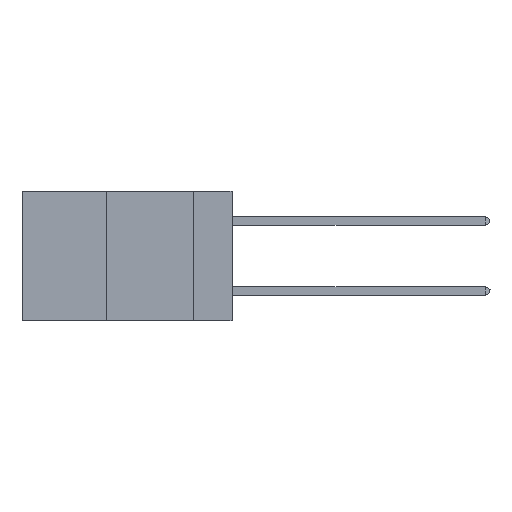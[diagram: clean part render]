
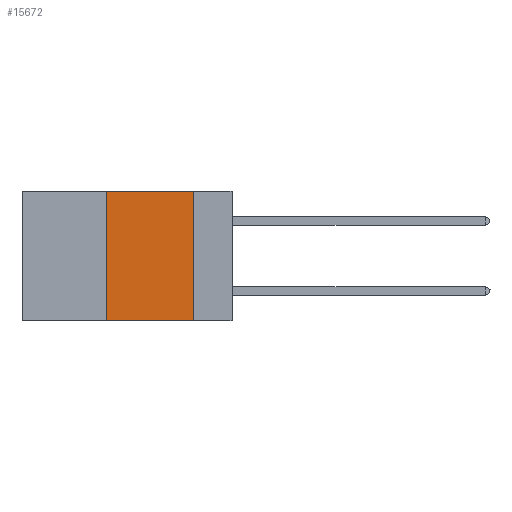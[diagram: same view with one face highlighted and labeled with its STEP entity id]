
A CAD part, left-side view. The second image highlights one B-rep face of the part: STEP entity #15672.
In plain terms, the highlighted planar face has unit normal (-1, 0, 0).
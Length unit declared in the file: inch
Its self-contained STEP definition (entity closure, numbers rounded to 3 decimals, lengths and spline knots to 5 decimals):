
#321 = PLANE ( 'NONE',  #1953 ) ;
#846 = VECTOR ( 'NONE', #3519, 39.37008 ) ;
#1703 = CARTESIAN_POINT ( 'NONE',  ( 0., 0.11, 0. ) ) ;
#1807 = VERTEX_POINT ( 'NONE', #18376 ) ;
#1953 = AXIS2_PLACEMENT_3D ( 'NONE', #6046, #10335, #5559 ) ;
#2399 = FACE_OUTER_BOUND ( 'NONE', #6142, .T. ) ;
#2814 = EDGE_CURVE ( 'NONE', #11081, #12556, #5614, .T. ) ;
#3041 = ORIENTED_EDGE ( 'NONE', *, *, #2814, .F. ) ;
#3519 = DIRECTION ( 'NONE',  ( 0., -1., 0. ) ) ;
#4513 = VECTOR ( 'NONE', #21857, 39.37008 ) ;
#4859 = LINE ( 'NONE', #13328, #4513 ) ;
#5559 = DIRECTION ( 'NONE',  ( 0., 0., -1. ) ) ;
#5614 = LINE ( 'NONE', #1703, #26925 ) ;
#5883 = ORIENTED_EDGE ( 'NONE', *, *, #22800, .F. ) ;
#6046 = CARTESIAN_POINT ( 'NONE',  ( 0., 0.6, 0. ) ) ;
#6142 = EDGE_LOOP ( 'NONE', ( #3041, #5883, #9761, #21176 ) ) ;
#7833 = DIRECTION ( 'NONE',  ( 0., 0., -1. ) ) ;
#9761 = ORIENTED_EDGE ( 'NONE', *, *, #15770, .F. ) ;
#10335 = DIRECTION ( 'NONE',  ( 1., 0., 0. ) ) ;
#11081 = VERTEX_POINT ( 'NONE', #18260 ) ;
#12556 = VERTEX_POINT ( 'NONE', #13640 ) ;
#12992 = EDGE_CURVE ( 'NONE', #1807, #12556, #4859, .T. ) ;
#13328 = CARTESIAN_POINT ( 'NONE',  ( 0., 0.6, -0.37 ) ) ;
#13640 = CARTESIAN_POINT ( 'NONE',  ( 0., 0.11, -0.37 ) ) ;
#14015 = LINE ( 'NONE', #19828, #14378 ) ;
#14378 = VECTOR ( 'NONE', #15191, 39.37008 ) ;
#15191 = DIRECTION ( 'NONE',  ( 0., 0., 1. ) ) ;
#15672 = ADVANCED_FACE ( 'NONE', ( #2399 ), #321, .F. ) ;
#15770 = EDGE_CURVE ( 'NONE', #1807, #16244, #14015, .T. ) ;
#16244 = VERTEX_POINT ( 'NONE', #20836 ) ;
#18260 = CARTESIAN_POINT ( 'NONE',  ( 0., 0.11, 0. ) ) ;
#18376 = CARTESIAN_POINT ( 'NONE',  ( 0., 0.36, -0.37 ) ) ;
#19828 = CARTESIAN_POINT ( 'NONE',  ( 0., 0.36, 0. ) ) ;
#20375 = CARTESIAN_POINT ( 'NONE',  ( 0., 0.6, 0. ) ) ;
#20836 = CARTESIAN_POINT ( 'NONE',  ( 0., 0.36, 0. ) ) ;
#21176 = ORIENTED_EDGE ( 'NONE', *, *, #12992, .T. ) ;
#21857 = DIRECTION ( 'NONE',  ( 0., -1., 0. ) ) ;
#22800 = EDGE_CURVE ( 'NONE', #16244, #11081, #24123, .T. ) ;
#24123 = LINE ( 'NONE', #20375, #846 ) ;
#26925 = VECTOR ( 'NONE', #7833, 39.37008 ) ;
